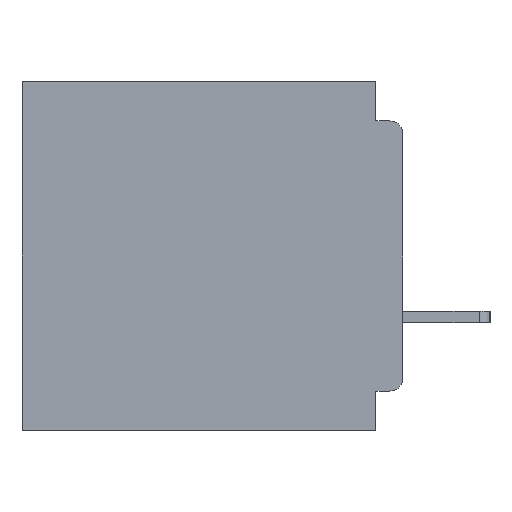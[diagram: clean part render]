
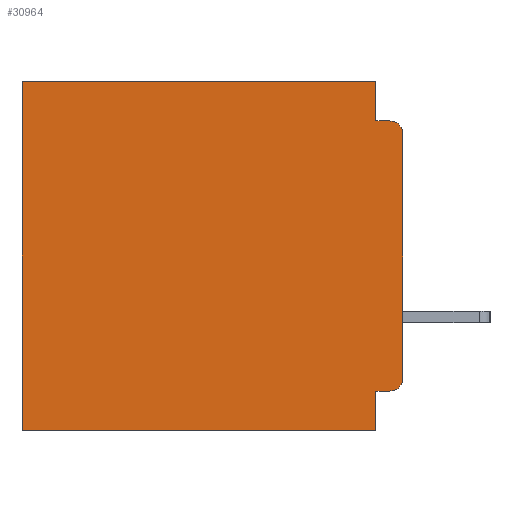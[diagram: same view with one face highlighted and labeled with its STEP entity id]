
A CAD part, left-side view. The second image highlights one B-rep face of the part: STEP entity #30964.
In plain terms, the highlighted planar face has unit normal (-1, 0, 0).
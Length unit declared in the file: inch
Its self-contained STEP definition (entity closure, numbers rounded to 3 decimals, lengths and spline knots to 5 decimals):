
#37 = CARTESIAN_POINT ( 'NONE',  ( 0.3, 0.437, -0.4 ) ) ;
#700 = EDGE_CURVE ( 'NONE', #3636, #5631, #14996, .T. ) ;
#2037 = DIRECTION ( 'NONE',  ( 0., 1., 0. ) ) ;
#2126 = ORIENTED_EDGE ( 'NONE', *, *, #20690, .F. ) ;
#2221 = ORIENTED_EDGE ( 'NONE', *, *, #14111, .T. ) ;
#3636 = VERTEX_POINT ( 'NONE', #16234 ) ;
#3637 = ORIENTED_EDGE ( 'NONE', *, *, #700, .F. ) ;
#3816 = ORIENTED_EDGE ( 'NONE', *, *, #36194, .F. ) ;
#4082 = EDGE_CURVE ( 'NONE', #45226, #13206, #44907, .T. ) ;
#4279 = DIRECTION ( 'NONE',  ( 0., 0., -1. ) ) ;
#4752 = VERTEX_POINT ( 'NONE', #9676 ) ;
#4997 = ORIENTED_EDGE ( 'NONE', *, *, #16071, .T. ) ;
#5217 = CARTESIAN_POINT ( 'NONE',  ( 0.3, 0.015, -0.34 ) ) ;
#5631 = VERTEX_POINT ( 'NONE', #31041 ) ;
#6128 = ORIENTED_EDGE ( 'NONE', *, *, #14074, .T. ) ;
#6491 = DIRECTION ( 'NONE',  ( -1., 0., 0. ) ) ;
#6820 = ORIENTED_EDGE ( 'NONE', *, *, #22788, .F. ) ;
#6972 = LINE ( 'NONE', #28138, #28038 ) ;
#7805 = ORIENTED_EDGE ( 'NONE', *, *, #28791, .F. ) ;
#7892 = ORIENTED_EDGE ( 'NONE', *, *, #19084, .F. ) ;
#8024 = ORIENTED_EDGE ( 'NONE', *, *, #4082, .T. ) ;
#8036 = VECTOR ( 'NONE', #39885, 39.37008 ) ;
#9641 = VECTOR ( 'NONE', #42167, 39.37008 ) ;
#9676 = CARTESIAN_POINT ( 'NONE',  ( 0.3, 0.437, 0. ) ) ;
#9717 = VERTEX_POINT ( 'NONE', #11946 ) ;
#10702 = CARTESIAN_POINT ( 'NONE',  ( 0.3, 0., -0.4 ) ) ;
#10950 = VECTOR ( 'NONE', #15222, 39.37008 ) ;
#11327 = VECTOR ( 'NONE', #11736, 39.37008 ) ;
#11689 = EDGE_LOOP ( 'NONE', ( #2126, #2221, #3637, #3816, #4997, #6128, #6820, #7805, #7892, #8024 ) ) ;
#11736 = DIRECTION ( 'NONE',  ( 0., 1., 0. ) ) ;
#11946 = CARTESIAN_POINT ( 'NONE',  ( 0.3, 0.031, -0.355 ) ) ;
#13044 = CARTESIAN_POINT ( 'NONE',  ( 0.3, 0.031, 0. ) ) ;
#13206 = VERTEX_POINT ( 'NONE', #19345 ) ;
#14074 = EDGE_CURVE ( 'NONE', #4752, #24774, #37748, .T. ) ;
#14111 = EDGE_CURVE ( 'NONE', #20042, #5631, #45260, .T. ) ;
#14996 = LINE ( 'NONE', #24527, #19670 ) ;
#15222 = DIRECTION ( 'NONE',  ( 0., 0., -1. ) ) ;
#15322 = CARTESIAN_POINT ( 'NONE',  ( 0.3, 0., 0. ) ) ;
#16071 = EDGE_CURVE ( 'NONE', #21654, #4752, #21255, .T. ) ;
#16234 = CARTESIAN_POINT ( 'NONE',  ( 0.3, 0.031, -0.045 ) ) ;
#18031 = PLANE ( 'NONE',  #22829 ) ;
#19084 = EDGE_CURVE ( 'NONE', #45226, #9717, #39330, .T. ) ;
#19345 = CARTESIAN_POINT ( 'NONE',  ( 0.3, 0., -0.34 ) ) ;
#19670 = VECTOR ( 'NONE', #46614, 39.37008 ) ;
#20042 = VERTEX_POINT ( 'NONE', #22421 ) ;
#20690 = EDGE_CURVE ( 'NONE', #20042, #13206, #25247, .T. ) ;
#20891 = LINE ( 'NONE', #22527, #10950 ) ;
#21115 = FACE_OUTER_BOUND ( 'NONE', #11689, .T. ) ;
#21255 = LINE ( 'NONE', #15322, #11327 ) ;
#21522 = DIRECTION ( 'NONE',  ( -1., 0., 0. ) ) ;
#21654 = VERTEX_POINT ( 'NONE', #13044 ) ;
#21949 = DIRECTION ( 'NONE',  ( 0., 0., -1. ) ) ;
#22051 = CARTESIAN_POINT ( 'NONE',  ( 0.3, 0.031, 0. ) ) ;
#22421 = CARTESIAN_POINT ( 'NONE',  ( 0.3, 0., -0.06 ) ) ;
#22527 = CARTESIAN_POINT ( 'NONE',  ( 0.3, 0.031, -0.4 ) ) ;
#22788 = EDGE_CURVE ( 'NONE', #34229, #24774, #6972, .T. ) ;
#22829 = AXIS2_PLACEMENT_3D ( 'NONE', #10702, #44170, #21949 ) ;
#24067 = VECTOR ( 'NONE', #44277, 39.37008 ) ;
#24527 = CARTESIAN_POINT ( 'NONE',  ( 0.3, 0., -0.045 ) ) ;
#24774 = VERTEX_POINT ( 'NONE', #37 ) ;
#25247 = LINE ( 'NONE', #25849, #24067 ) ;
#25849 = CARTESIAN_POINT ( 'NONE',  ( 0.3, 0., -0.4 ) ) ;
#28038 = VECTOR ( 'NONE', #2037, 39.37008 ) ;
#28138 = CARTESIAN_POINT ( 'NONE',  ( 0.3, 0., -0.4 ) ) ;
#28295 = AXIS2_PLACEMENT_3D ( 'NONE', #5217, #6491, #4279 ) ;
#28791 = EDGE_CURVE ( 'NONE', #9717, #34229, #20891, .T. ) ;
#29609 = DIRECTION ( 'NONE',  ( 0., 0., -1. ) ) ;
#30964 = ADVANCED_FACE ( 'NONE', ( #21115 ), #18031, .F. ) ;
#31041 = CARTESIAN_POINT ( 'NONE',  ( 0.3, 0.015, -0.045 ) ) ;
#34229 = VERTEX_POINT ( 'NONE', #36846 ) ;
#34668 = VECTOR ( 'NONE', #29609, 39.37008 ) ;
#35826 = LINE ( 'NONE', #22051, #34668 ) ;
#36162 = CARTESIAN_POINT ( 'NONE',  ( 0.3, 0.437, -0.4 ) ) ;
#36194 = EDGE_CURVE ( 'NONE', #21654, #3636, #35826, .T. ) ;
#36846 = CARTESIAN_POINT ( 'NONE',  ( 0.3, 0.031, -0.4 ) ) ;
#37748 = LINE ( 'NONE', #36162, #8036 ) ;
#38453 = CARTESIAN_POINT ( 'NONE',  ( 0.3, 0., -0.355 ) ) ;
#39330 = LINE ( 'NONE', #38453, #9641 ) ;
#39885 = DIRECTION ( 'NONE',  ( 0., 0., -1. ) ) ;
#42167 = DIRECTION ( 'NONE',  ( 0., 1., 0. ) ) ;
#43750 = CARTESIAN_POINT ( 'NONE',  ( 0.3, 0.015, -0.06 ) ) ;
#44170 = DIRECTION ( 'NONE',  ( 1., 0., 0. ) ) ;
#44191 = CARTESIAN_POINT ( 'NONE',  ( 0.3, 0.015, -0.355 ) ) ;
#44277 = DIRECTION ( 'NONE',  ( 0., 0., -1. ) ) ;
#44907 = CIRCLE ( 'NONE', #28295, 0.015 ) ;
#45226 = VERTEX_POINT ( 'NONE', #44191 ) ;
#45260 = CIRCLE ( 'NONE', #46282, 0.015 ) ;
#46282 = AXIS2_PLACEMENT_3D ( 'NONE', #43750, #21522, #47457 ) ;
#46614 = DIRECTION ( 'NONE',  ( 0., -1., 0. ) ) ;
#47457 = DIRECTION ( 'NONE',  ( 0., 0., -1. ) ) ;
